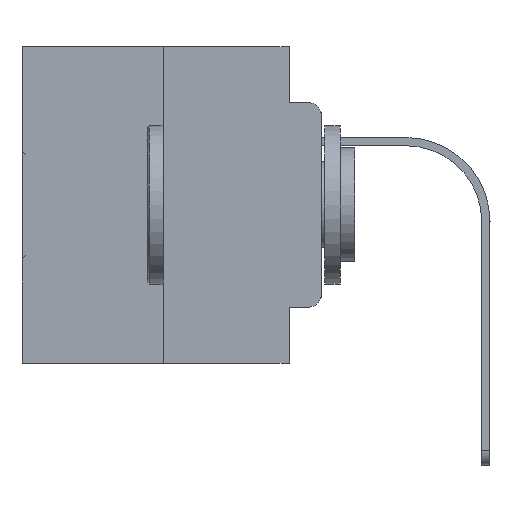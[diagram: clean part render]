
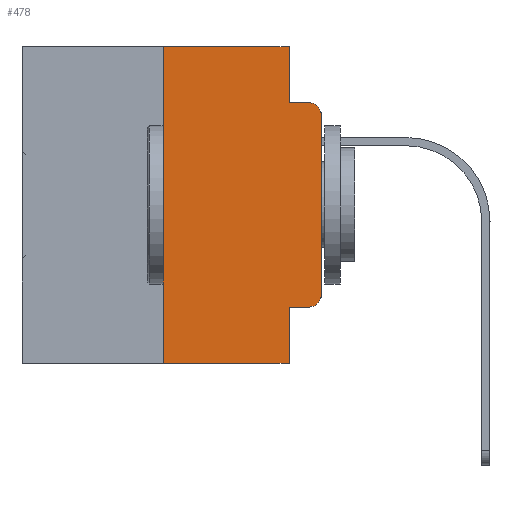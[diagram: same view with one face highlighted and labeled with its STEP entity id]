
A CAD part, left-side view. The second image highlights one B-rep face of the part: STEP entity #478.
In plain terms, the highlighted planar face has unit normal (-1, 0, 0).
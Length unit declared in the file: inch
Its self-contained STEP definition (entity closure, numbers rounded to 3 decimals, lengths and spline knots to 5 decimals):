
#478 = ADVANCED_FACE ( 'NONE', ( #26689 ), #28996, .F. ) ;
#1105 = DIRECTION ( 'NONE',  ( -1., 0., 0. ) ) ;
#1240 = DIRECTION ( 'NONE',  ( 0., 0., -1. ) ) ;
#1321 = CARTESIAN_POINT ( 'NONE',  ( 0., 0.473, -0.5 ) ) ;
#1326 = DIRECTION ( 'NONE',  ( 0., 0., -1. ) ) ;
#1514 = ORIENTED_EDGE ( 'NONE', *, *, #24106, .T. ) ;
#1774 = CARTESIAN_POINT ( 'NONE',  ( 0., 0.473, 0. ) ) ;
#1878 = CIRCLE ( 'NONE', #31556, 0.02 ) ;
#1935 = EDGE_CURVE ( 'NONE', #29960, #11490, #11969, .T. ) ;
#2465 = VECTOR ( 'NONE', #31692, 39.37008 ) ;
#2731 = CIRCLE ( 'NONE', #25534, 0.02 ) ;
#2890 = VERTEX_POINT ( 'NONE', #12504 ) ;
#2923 = EDGE_CURVE ( 'NONE', #18005, #12472, #10981, .T. ) ;
#2924 = EDGE_CURVE ( 'NONE', #12472, #26056, #3340, .T. ) ;
#3340 = LINE ( 'NONE', #26089, #28528 ) ;
#3490 = ORIENTED_EDGE ( 'NONE', *, *, #11677, .T. ) ;
#3797 = CARTESIAN_POINT ( 'NONE',  ( 0., 0., -0.3915 ) ) ;
#3905 = DIRECTION ( 'NONE',  ( -1., 0., 0. ) ) ;
#3915 = VECTOR ( 'NONE', #29796, 39.37008 ) ;
#5627 = ORIENTED_EDGE ( 'NONE', *, *, #2924, .F. ) ;
#5831 = CARTESIAN_POINT ( 'NONE',  ( 0., 0.473, 0. ) ) ;
#6083 = DIRECTION ( 'NONE',  ( 0., 0., -1. ) ) ;
#6281 = EDGE_CURVE ( 'NONE', #24269, #30083, #2731, .T. ) ;
#6473 = ORIENTED_EDGE ( 'NONE', *, *, #31703, .T. ) ;
#6671 = CARTESIAN_POINT ( 'NONE',  ( 0., 0.051, -0.0885 ) ) ;
#6805 = VECTOR ( 'NONE', #31129, 39.37008 ) ;
#8243 = CARTESIAN_POINT ( 'NONE',  ( 0., 0., 0. ) ) ;
#8915 = AXIS2_PLACEMENT_3D ( 'NONE', #1774, #24370, #21730 ) ;
#9267 = ORIENTED_EDGE ( 'NONE', *, *, #10541, .F. ) ;
#10541 = EDGE_CURVE ( 'NONE', #26056, #2890, #19450, .T. ) ;
#10981 = LINE ( 'NONE', #5831, #25881 ) ;
#11074 = LINE ( 'NONE', #8243, #6805 ) ;
#11110 = EDGE_CURVE ( 'NONE', #30519, #11490, #12054, .T. ) ;
#11323 = DIRECTION ( 'NONE',  ( 0., -1., 0. ) ) ;
#11377 = LINE ( 'NONE', #21507, #18033 ) ;
#11490 = VERTEX_POINT ( 'NONE', #19492 ) ;
#11677 = EDGE_CURVE ( 'NONE', #30519, #24269, #27905, .T. ) ;
#11969 = LINE ( 'NONE', #1321, #2465 ) ;
#12054 = LINE ( 'NONE', #32269, #3915 ) ;
#12264 = CARTESIAN_POINT ( 'NONE',  ( 0., 0.051, 0. ) ) ;
#12472 = VERTEX_POINT ( 'NONE', #12264 ) ;
#12504 = CARTESIAN_POINT ( 'NONE',  ( 0., 0.02, -0.0885 ) ) ;
#12987 = CARTESIAN_POINT ( 'NONE',  ( 0., 0.051, -0.4115 ) ) ;
#13514 = VECTOR ( 'NONE', #17476, 39.37008 ) ;
#13986 = ORIENTED_EDGE ( 'NONE', *, *, #2923, .F. ) ;
#14355 = VERTEX_POINT ( 'NONE', #30237 ) ;
#15586 = CARTESIAN_POINT ( 'NONE',  ( 0., 0.25, -0.5 ) ) ;
#17476 = DIRECTION ( 'NONE',  ( 0., -1., 0. ) ) ;
#18005 = VERTEX_POINT ( 'NONE', #32288 ) ;
#18033 = VECTOR ( 'NONE', #26297, 39.37008 ) ;
#18937 = CARTESIAN_POINT ( 'NONE',  ( 0., 0.051, -0.0885 ) ) ;
#19450 = LINE ( 'NONE', #18937, #29860 ) ;
#19492 = CARTESIAN_POINT ( 'NONE',  ( 0., 0.051, -0.5 ) ) ;
#21507 = CARTESIAN_POINT ( 'NONE',  ( 0., 0.25, 0. ) ) ;
#21730 = DIRECTION ( 'NONE',  ( 0., 0., -1. ) ) ;
#21748 = ORIENTED_EDGE ( 'NONE', *, *, #22766, .F. ) ;
#22766 = EDGE_CURVE ( 'NONE', #29960, #18005, #11377, .T. ) ;
#23835 = ORIENTED_EDGE ( 'NONE', *, *, #6281, .T. ) ;
#24106 = EDGE_CURVE ( 'NONE', #14355, #2890, #1878, .T. ) ;
#24247 = DIRECTION ( 'NONE',  ( 0., -1., 0. ) ) ;
#24269 = VERTEX_POINT ( 'NONE', #24814 ) ;
#24370 = DIRECTION ( 'NONE',  ( 1., 0., 0. ) ) ;
#24635 = CARTESIAN_POINT ( 'NONE',  ( 0., 0.051, -0.4115 ) ) ;
#24814 = CARTESIAN_POINT ( 'NONE',  ( 0., 0.02, -0.4115 ) ) ;
#25534 = AXIS2_PLACEMENT_3D ( 'NONE', #30813, #1105, #6083 ) ;
#25843 = ORIENTED_EDGE ( 'NONE', *, *, #11110, .F. ) ;
#25881 = VECTOR ( 'NONE', #11323, 39.37008 ) ;
#26056 = VERTEX_POINT ( 'NONE', #6671 ) ;
#26089 = CARTESIAN_POINT ( 'NONE',  ( 0., 0.051, 0. ) ) ;
#26297 = DIRECTION ( 'NONE',  ( 0., 0., 1. ) ) ;
#26689 = FACE_OUTER_BOUND ( 'NONE', #28792, .T. ) ;
#27890 = ORIENTED_EDGE ( 'NONE', *, *, #1935, .T. ) ;
#27905 = LINE ( 'NONE', #12987, #13514 ) ;
#28528 = VECTOR ( 'NONE', #1326, 39.37008 ) ;
#28792 = EDGE_LOOP ( 'NONE', ( #6473, #1514, #9267, #5627, #13986, #21748, #27890, #25843, #3490, #23835 ) ) ;
#28996 = PLANE ( 'NONE',  #8915 ) ;
#29796 = DIRECTION ( 'NONE',  ( 0., 0., -1. ) ) ;
#29860 = VECTOR ( 'NONE', #24247, 39.37008 ) ;
#29960 = VERTEX_POINT ( 'NONE', #15586 ) ;
#30083 = VERTEX_POINT ( 'NONE', #3797 ) ;
#30237 = CARTESIAN_POINT ( 'NONE',  ( 0., 0., -0.1085 ) ) ;
#30519 = VERTEX_POINT ( 'NONE', #24635 ) ;
#30813 = CARTESIAN_POINT ( 'NONE',  ( 0., 0.02, -0.3915 ) ) ;
#31129 = DIRECTION ( 'NONE',  ( 0., 0., 1. ) ) ;
#31556 = AXIS2_PLACEMENT_3D ( 'NONE', #31768, #3905, #1240 ) ;
#31692 = DIRECTION ( 'NONE',  ( 0., -1., 0. ) ) ;
#31703 = EDGE_CURVE ( 'NONE', #30083, #14355, #11074, .T. ) ;
#31768 = CARTESIAN_POINT ( 'NONE',  ( 0., 0.02, -0.1085 ) ) ;
#32269 = CARTESIAN_POINT ( 'NONE',  ( 0., 0.051, 0. ) ) ;
#32288 = CARTESIAN_POINT ( 'NONE',  ( 0., 0.25, 0. ) ) ;
